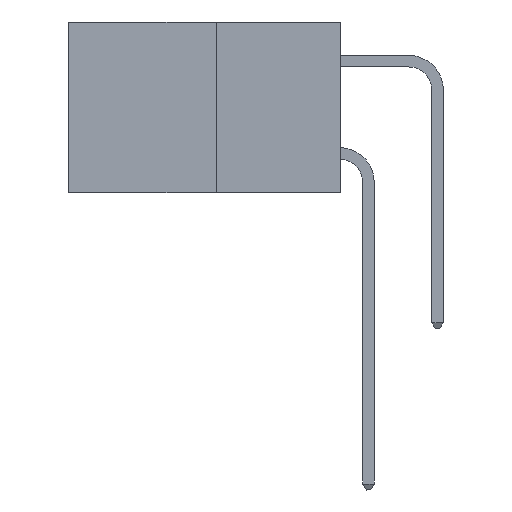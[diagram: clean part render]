
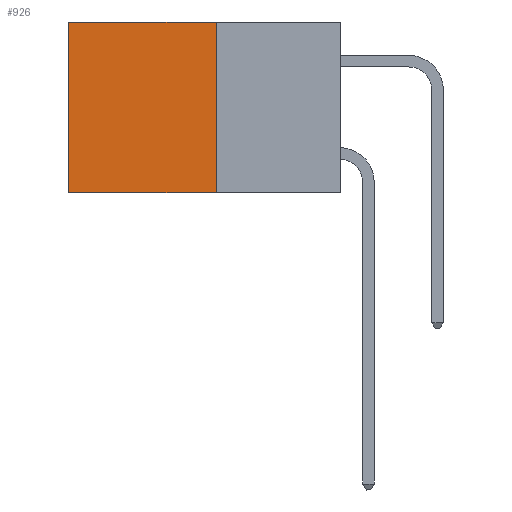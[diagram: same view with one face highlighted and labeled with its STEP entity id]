
A CAD part, left-side view. The second image highlights one B-rep face of the part: STEP entity #926.
In plain terms, the highlighted planar face has unit normal (-1, 0, 0).
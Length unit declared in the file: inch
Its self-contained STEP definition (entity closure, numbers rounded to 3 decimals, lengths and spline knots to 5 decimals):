
#926 = ADVANCED_FACE ( 'NONE', ( #7212 ), #11363, .F. ) ;
#1214 = LINE ( 'NONE', #1888, #17058 ) ;
#1649 = VECTOR ( 'NONE', #14155, 39.37008 ) ;
#1888 = CARTESIAN_POINT ( 'NONE',  ( 0.277, 0.27, 0. ) ) ;
#3579 = ORIENTED_EDGE ( 'NONE', *, *, #13576, .F. ) ;
#3995 = DIRECTION ( 'NONE',  ( 0., 1., 0. ) ) ;
#5237 = VERTEX_POINT ( 'NONE', #12268 ) ;
#5499 = VECTOR ( 'NONE', #18192, 39.37008 ) ;
#6105 = EDGE_CURVE ( 'NONE', #14805, #25233, #10399, .T. ) ;
#6545 = LINE ( 'NONE', #20207, #1649 ) ;
#7212 = FACE_OUTER_BOUND ( 'NONE', #10082, .T. ) ;
#7965 = CARTESIAN_POINT ( 'NONE',  ( 0.277, 0.27, -0.37 ) ) ;
#9319 = ORIENTED_EDGE ( 'NONE', *, *, #15617, .T. ) ;
#10010 = CARTESIAN_POINT ( 'NONE',  ( 0.277, 0.59, -0.37 ) ) ;
#10082 = EDGE_LOOP ( 'NONE', ( #25244, #3579, #19582, #9319 ) ) ;
#10213 = CARTESIAN_POINT ( 'NONE',  ( 0.277, 0.59, -0.37 ) ) ;
#10399 = LINE ( 'NONE', #18439, #5499 ) ;
#10983 = LINE ( 'NONE', #10213, #15755 ) ;
#11363 = PLANE ( 'NONE',  #14433 ) ;
#12268 = CARTESIAN_POINT ( 'NONE',  ( 0.277, 0.59, 0. ) ) ;
#13552 = VERTEX_POINT ( 'NONE', #10010 ) ;
#13576 = EDGE_CURVE ( 'NONE', #25233, #13552, #6545, .T. ) ;
#14155 = DIRECTION ( 'NONE',  ( 0., 1., 0. ) ) ;
#14433 = AXIS2_PLACEMENT_3D ( 'NONE', #20799, #23512, #20331 ) ;
#14805 = VERTEX_POINT ( 'NONE', #18077 ) ;
#15617 = EDGE_CURVE ( 'NONE', #14805, #5237, #1214, .T. ) ;
#15755 = VECTOR ( 'NONE', #16374, 39.37008 ) ;
#16374 = DIRECTION ( 'NONE',  ( 0., 0., -1. ) ) ;
#17058 = VECTOR ( 'NONE', #3995, 39.37008 ) ;
#18077 = CARTESIAN_POINT ( 'NONE',  ( 0.277, 0.27, 0. ) ) ;
#18192 = DIRECTION ( 'NONE',  ( 0., 0., -1. ) ) ;
#18439 = CARTESIAN_POINT ( 'NONE',  ( 0.277, 0.27, -0.37 ) ) ;
#19582 = ORIENTED_EDGE ( 'NONE', *, *, #6105, .F. ) ;
#20207 = CARTESIAN_POINT ( 'NONE',  ( 0.277, 0.27, -0.37 ) ) ;
#20331 = DIRECTION ( 'NONE',  ( 0., 0., -1. ) ) ;
#20799 = CARTESIAN_POINT ( 'NONE',  ( 0.277, 0.27, -0.37 ) ) ;
#23512 = DIRECTION ( 'NONE',  ( 1., 0., 0. ) ) ;
#25233 = VERTEX_POINT ( 'NONE', #7965 ) ;
#25244 = ORIENTED_EDGE ( 'NONE', *, *, #26196, .T. ) ;
#26196 = EDGE_CURVE ( 'NONE', #5237, #13552, #10983, .T. ) ;
